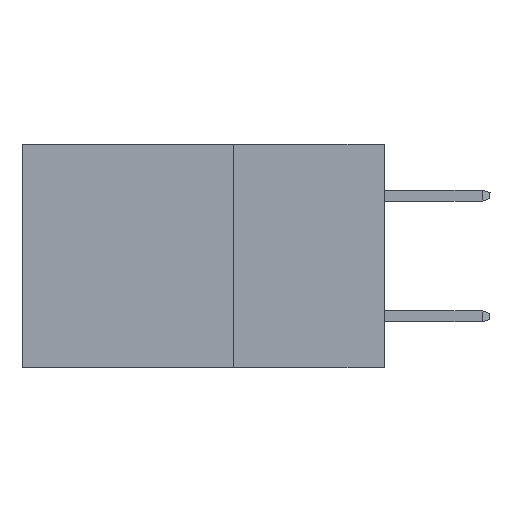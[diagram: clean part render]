
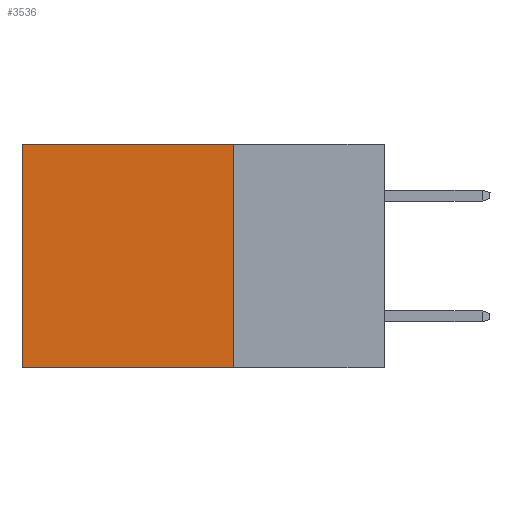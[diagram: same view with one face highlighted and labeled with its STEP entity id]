
A CAD part, left-side view. The second image highlights one B-rep face of the part: STEP entity #3536.
In plain terms, the highlighted planar face has unit normal (-1, 0, 0).
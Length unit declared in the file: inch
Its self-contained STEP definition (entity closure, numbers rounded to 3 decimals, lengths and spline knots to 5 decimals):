
#462 = DIRECTION ( 'NONE',  ( 0., 0., -1. ) ) ;
#960 = VERTEX_POINT ( 'NONE', #10107 ) ;
#1128 = DIRECTION ( 'NONE',  ( 0., 0., -1. ) ) ;
#1374 = ORIENTED_EDGE ( 'NONE', *, *, #3042, .F. ) ;
#1943 = VERTEX_POINT ( 'NONE', #3994 ) ;
#2281 = VERTEX_POINT ( 'NONE', #7786 ) ;
#2672 = ORIENTED_EDGE ( 'NONE', *, *, #10514, .T. ) ;
#2717 = EDGE_CURVE ( 'NONE', #960, #3893, #8424, .T. ) ;
#2806 = CARTESIAN_POINT ( 'NONE',  ( 0.298, 0.25, -0.37 ) ) ;
#3042 = EDGE_CURVE ( 'NONE', #2281, #960, #8837, .T. ) ;
#3113 = VECTOR ( 'NONE', #462, 39.37008 ) ;
#3536 = ADVANCED_FACE ( 'NONE', ( #6620 ), #4953, .F. ) ;
#3893 = VERTEX_POINT ( 'NONE', #8037 ) ;
#3994 = CARTESIAN_POINT ( 'NONE',  ( 0.298, 0.6, 0. ) ) ;
#4953 = PLANE ( 'NONE',  #7302 ) ;
#5104 = DIRECTION ( 'NONE',  ( 0., 0., -1. ) ) ;
#6620 = FACE_OUTER_BOUND ( 'NONE', #8137, .T. ) ;
#7153 = EDGE_CURVE ( 'NONE', #2281, #1943, #10839, .T. ) ;
#7302 = AXIS2_PLACEMENT_3D ( 'NONE', #8596, #10424, #1128 ) ;
#7776 = CARTESIAN_POINT ( 'NONE',  ( 0.298, 0.6, 0. ) ) ;
#7786 = CARTESIAN_POINT ( 'NONE',  ( 0.298, 0.25, 0. ) ) ;
#8037 = CARTESIAN_POINT ( 'NONE',  ( 0.298, 0.6, -0.37 ) ) ;
#8137 = EDGE_LOOP ( 'NONE', ( #2672, #10856, #1374, #8616 ) ) ;
#8227 = DIRECTION ( 'NONE',  ( 0., 1., 0. ) ) ;
#8424 = LINE ( 'NONE', #2806, #11127 ) ;
#8490 = LINE ( 'NONE', #7776, #3113 ) ;
#8596 = CARTESIAN_POINT ( 'NONE',  ( 0.298, 0.25, 0. ) ) ;
#8616 = ORIENTED_EDGE ( 'NONE', *, *, #7153, .T. ) ;
#8837 = LINE ( 'NONE', #11472, #9039 ) ;
#9039 = VECTOR ( 'NONE', #5104, 39.37008 ) ;
#9257 = DIRECTION ( 'NONE',  ( 0., 1., 0. ) ) ;
#10107 = CARTESIAN_POINT ( 'NONE',  ( 0.298, 0.25, -0.37 ) ) ;
#10412 = VECTOR ( 'NONE', #8227, 39.37008 ) ;
#10424 = DIRECTION ( 'NONE',  ( 1., 0., 0. ) ) ;
#10514 = EDGE_CURVE ( 'NONE', #1943, #3893, #8490, .T. ) ;
#10839 = LINE ( 'NONE', #11777, #10412 ) ;
#10856 = ORIENTED_EDGE ( 'NONE', *, *, #2717, .F. ) ;
#11127 = VECTOR ( 'NONE', #9257, 39.37008 ) ;
#11472 = CARTESIAN_POINT ( 'NONE',  ( 0.298, 0.25, 0. ) ) ;
#11777 = CARTESIAN_POINT ( 'NONE',  ( 0.298, 0.25, 0. ) ) ;
